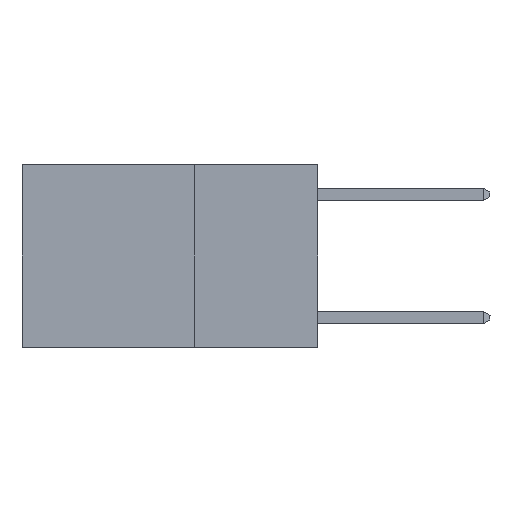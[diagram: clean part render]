
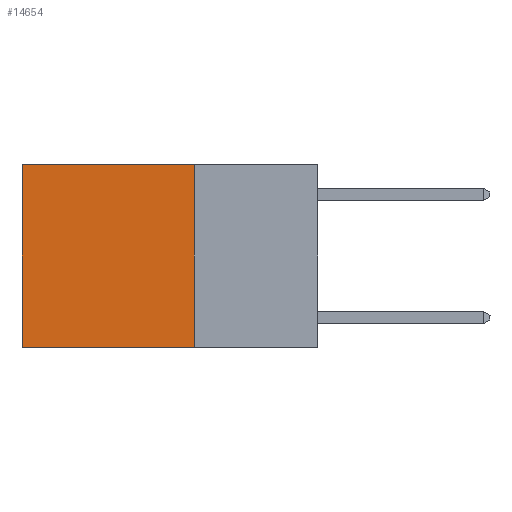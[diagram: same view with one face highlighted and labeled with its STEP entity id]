
A CAD part, left-side view. The second image highlights one B-rep face of the part: STEP entity #14654.
In plain terms, the highlighted planar face has unit normal (-1, 0, 0).
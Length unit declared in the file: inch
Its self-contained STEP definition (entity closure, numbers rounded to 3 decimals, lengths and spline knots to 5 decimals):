
#1927 = CARTESIAN_POINT ( 'NONE',  ( 0.2625, 0.25, 0. ) ) ;
#2003 = CARTESIAN_POINT ( 'NONE',  ( 0.2625, 0.25, 0. ) ) ;
#2051 = VERTEX_POINT ( 'NONE', #2003 ) ;
#2691 = EDGE_LOOP ( 'NONE', ( #23382, #21013, #27270, #10139 ) ) ;
#4062 = DIRECTION ( 'NONE',  ( 0., 0., -1. ) ) ;
#4271 = CARTESIAN_POINT ( 'NONE',  ( 0.2625, 0.6, 0. ) ) ;
#4886 = AXIS2_PLACEMENT_3D ( 'NONE', #1927, #16788, #4062 ) ;
#5453 = CARTESIAN_POINT ( 'NONE',  ( 0.2625, 0.25, -0.37 ) ) ;
#5690 = DIRECTION ( 'NONE',  ( 0., 0., -1. ) ) ;
#6133 = FACE_OUTER_BOUND ( 'NONE', #2691, .T. ) ;
#6858 = LINE ( 'NONE', #11903, #22403 ) ;
#7867 = CARTESIAN_POINT ( 'NONE',  ( 0.2625, 0.25, -0.37 ) ) ;
#9153 = EDGE_CURVE ( 'NONE', #18417, #15527, #13411, .T. ) ;
#9619 = LINE ( 'NONE', #15161, #23512 ) ;
#9684 = DIRECTION ( 'NONE',  ( 0., 1., 0. ) ) ;
#10139 = ORIENTED_EDGE ( 'NONE', *, *, #13800, .T. ) ;
#10319 = VECTOR ( 'NONE', #22370, 39.37008 ) ;
#11903 = CARTESIAN_POINT ( 'NONE',  ( 0.2625, 0.25, 0. ) ) ;
#13077 = VERTEX_POINT ( 'NONE', #7867 ) ;
#13411 = LINE ( 'NONE', #18398, #21007 ) ;
#13800 = EDGE_CURVE ( 'NONE', #2051, #18417, #6858, .T. ) ;
#14654 = ADVANCED_FACE ( 'NONE', ( #6133 ), #23040, .F. ) ;
#15161 = CARTESIAN_POINT ( 'NONE',  ( 0.2625, 0.25, 0. ) ) ;
#15527 = VERTEX_POINT ( 'NONE', #26737 ) ;
#16788 = DIRECTION ( 'NONE',  ( 1., 0., 0. ) ) ;
#17429 = EDGE_CURVE ( 'NONE', #13077, #15527, #26196, .T. ) ;
#18398 = CARTESIAN_POINT ( 'NONE',  ( 0.2625, 0.6, 0. ) ) ;
#18417 = VERTEX_POINT ( 'NONE', #4271 ) ;
#19012 = EDGE_CURVE ( 'NONE', #2051, #13077, #9619, .T. ) ;
#21007 = VECTOR ( 'NONE', #5690, 39.37008 ) ;
#21013 = ORIENTED_EDGE ( 'NONE', *, *, #17429, .F. ) ;
#21693 = DIRECTION ( 'NONE',  ( 0., 0., -1. ) ) ;
#22370 = DIRECTION ( 'NONE',  ( 0., 1., 0. ) ) ;
#22403 = VECTOR ( 'NONE', #9684, 39.37008 ) ;
#23040 = PLANE ( 'NONE',  #4886 ) ;
#23382 = ORIENTED_EDGE ( 'NONE', *, *, #9153, .T. ) ;
#23512 = VECTOR ( 'NONE', #21693, 39.37008 ) ;
#26196 = LINE ( 'NONE', #5453, #10319 ) ;
#26737 = CARTESIAN_POINT ( 'NONE',  ( 0.2625, 0.6, -0.37 ) ) ;
#27270 = ORIENTED_EDGE ( 'NONE', *, *, #19012, .F. ) ;
